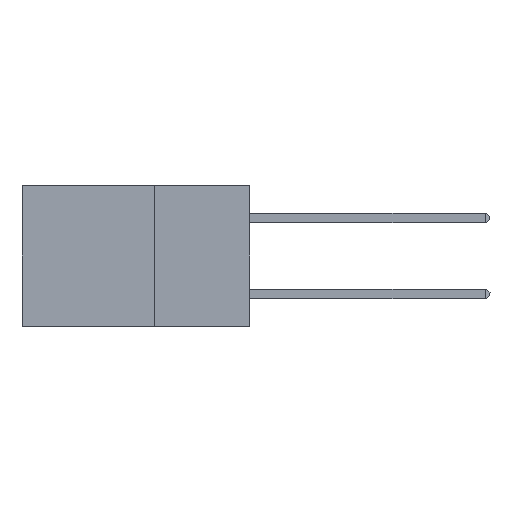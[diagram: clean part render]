
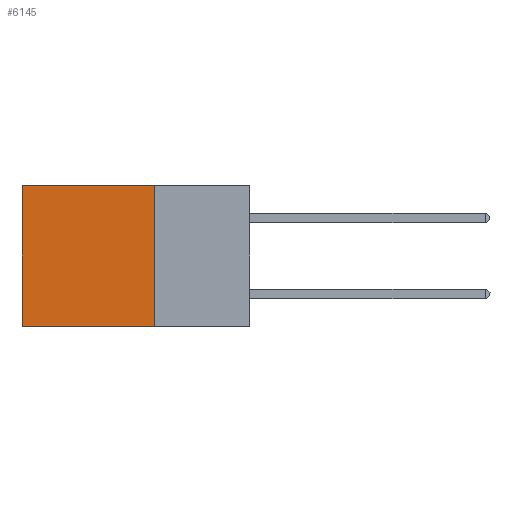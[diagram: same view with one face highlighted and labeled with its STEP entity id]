
A CAD part, left-side view. The second image highlights one B-rep face of the part: STEP entity #6145.
In plain terms, the highlighted planar face has unit normal (-1, 0, 0).
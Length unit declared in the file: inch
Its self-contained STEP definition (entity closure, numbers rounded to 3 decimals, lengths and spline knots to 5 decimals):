
#457 = LINE ( 'NONE', #968, #5275 ) ;
#843 = DIRECTION ( 'NONE',  ( 0., 1., 0. ) ) ;
#968 = CARTESIAN_POINT ( 'NONE',  ( 0.2875, 0.6, 0. ) ) ;
#1369 = DIRECTION ( 'NONE',  ( 0., 0., -1. ) ) ;
#1488 = LINE ( 'NONE', #5390, #12869 ) ;
#1509 = EDGE_LOOP ( 'NONE', ( #1776, #8119, #14418, #12331 ) ) ;
#1558 = AXIS2_PLACEMENT_3D ( 'NONE', #4487, #11432, #12533 ) ;
#1776 = ORIENTED_EDGE ( 'NONE', *, *, #12795, .T. ) ;
#1930 = CARTESIAN_POINT ( 'NONE',  ( 0.2875, 0.25, 0. ) ) ;
#3046 = EDGE_CURVE ( 'NONE', #8315, #8158, #8821, .T. ) ;
#3092 = VERTEX_POINT ( 'NONE', #11345 ) ;
#3136 = VECTOR ( 'NONE', #8884, 39.37008 ) ;
#4049 = FACE_OUTER_BOUND ( 'NONE', #1509, .T. ) ;
#4145 = CARTESIAN_POINT ( 'NONE',  ( 0.2875, 0.25, -0.37 ) ) ;
#4487 = CARTESIAN_POINT ( 'NONE',  ( 0.2875, 0.25, 0. ) ) ;
#5275 = VECTOR ( 'NONE', #10207, 39.37008 ) ;
#5390 = CARTESIAN_POINT ( 'NONE',  ( 0.2875, 0.25, 0. ) ) ;
#6145 = ADVANCED_FACE ( 'NONE', ( #4049 ), #12429, .F. ) ;
#6669 = CARTESIAN_POINT ( 'NONE',  ( 0.2875, 0.25, -0.37 ) ) ;
#7451 = VECTOR ( 'NONE', #1369, 39.37008 ) ;
#8119 = ORIENTED_EDGE ( 'NONE', *, *, #3046, .F. ) ;
#8158 = VERTEX_POINT ( 'NONE', #11190 ) ;
#8315 = VERTEX_POINT ( 'NONE', #4145 ) ;
#8821 = LINE ( 'NONE', #6669, #3136 ) ;
#8884 = DIRECTION ( 'NONE',  ( 0., 1., 0. ) ) ;
#10207 = DIRECTION ( 'NONE',  ( 0., 0., -1. ) ) ;
#10356 = CARTESIAN_POINT ( 'NONE',  ( 0.2875, 0.25, 0. ) ) ;
#11019 = EDGE_CURVE ( 'NONE', #13844, #8315, #14535, .T. ) ;
#11190 = CARTESIAN_POINT ( 'NONE',  ( 0.2875, 0.6, -0.37 ) ) ;
#11345 = CARTESIAN_POINT ( 'NONE',  ( 0.2875, 0.6, 0. ) ) ;
#11432 = DIRECTION ( 'NONE',  ( 1., 0., 0. ) ) ;
#12331 = ORIENTED_EDGE ( 'NONE', *, *, #13909, .T. ) ;
#12429 = PLANE ( 'NONE',  #1558 ) ;
#12533 = DIRECTION ( 'NONE',  ( 0., 0., -1. ) ) ;
#12795 = EDGE_CURVE ( 'NONE', #3092, #8158, #457, .T. ) ;
#12869 = VECTOR ( 'NONE', #843, 39.37008 ) ;
#13844 = VERTEX_POINT ( 'NONE', #1930 ) ;
#13909 = EDGE_CURVE ( 'NONE', #13844, #3092, #1488, .T. ) ;
#14418 = ORIENTED_EDGE ( 'NONE', *, *, #11019, .F. ) ;
#14535 = LINE ( 'NONE', #10356, #7451 ) ;
